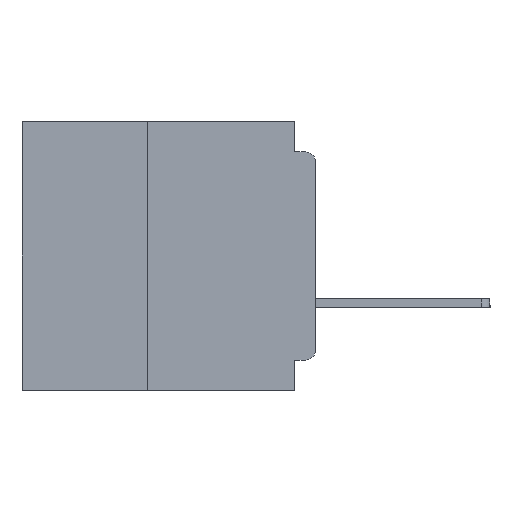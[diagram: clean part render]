
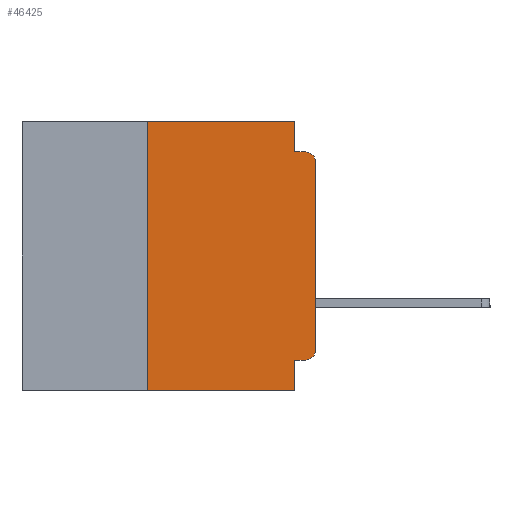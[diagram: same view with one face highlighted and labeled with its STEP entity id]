
A CAD part, left-side view. The second image highlights one B-rep face of the part: STEP entity #46425.
In plain terms, the highlighted planar face has unit normal (-1, 0, 0).
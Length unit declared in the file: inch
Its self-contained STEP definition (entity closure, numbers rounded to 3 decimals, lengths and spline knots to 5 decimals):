
#158 = VERTEX_POINT ( 'NONE', #44813 ) ;
#260 = ORIENTED_EDGE ( 'NONE', *, *, #31546, .T. ) ;
#1217 = CARTESIAN_POINT ( 'NONE',  ( 0., 0.437, 0. ) ) ;
#1366 = CARTESIAN_POINT ( 'NONE',  ( 0., 0., 0. ) ) ;
#1409 = DIRECTION ( 'NONE',  ( 0., 0., -1. ) ) ;
#1704 = VERTEX_POINT ( 'NONE', #16369 ) ;
#2099 = VECTOR ( 'NONE', #24303, 39.37008 ) ;
#3854 = VERTEX_POINT ( 'NONE', #15556 ) ;
#4200 = EDGE_CURVE ( 'NONE', #3854, #1704, #4926, .T. ) ;
#4202 = CARTESIAN_POINT ( 'NONE',  ( 0., 0.015, -0.06 ) ) ;
#4507 = DIRECTION ( 'NONE',  ( -1., 0., 0. ) ) ;
#4753 = DIRECTION ( 'NONE',  ( 0., 1., 0. ) ) ;
#4926 = LINE ( 'NONE', #34712, #16187 ) ;
#4936 = LINE ( 'NONE', #13848, #48570 ) ;
#5078 = CARTESIAN_POINT ( 'NONE',  ( 0., 0.015, -0.045 ) ) ;
#5503 = DIRECTION ( 'NONE',  ( 0., -1., 0. ) ) ;
#5647 = DIRECTION ( 'NONE',  ( 0., 0., 1. ) ) ;
#6201 = LINE ( 'NONE', #14201, #29228 ) ;
#7876 = VECTOR ( 'NONE', #4753, 39.37008 ) ;
#8481 = DIRECTION ( 'NONE',  ( 0., 0., -1. ) ) ;
#8859 = EDGE_CURVE ( 'NONE', #26395, #14210, #9221, .T. ) ;
#9221 = LINE ( 'NONE', #1366, #29024 ) ;
#9408 = DIRECTION ( 'NONE',  ( 0., 0., -1. ) ) ;
#10804 = CARTESIAN_POINT ( 'NONE',  ( 0., 0.25, -0.4 ) ) ;
#11711 = CARTESIAN_POINT ( 'NONE',  ( 0., 0., -0.045 ) ) ;
#11848 = AXIS2_PLACEMENT_3D ( 'NONE', #29822, #4507, #34080 ) ;
#12430 = CARTESIAN_POINT ( 'NONE',  ( 0., 0., -0.06 ) ) ;
#13848 = CARTESIAN_POINT ( 'NONE',  ( 0., 0.25, -0.4 ) ) ;
#14106 = CIRCLE ( 'NONE', #11848, 0.015 ) ;
#14201 = CARTESIAN_POINT ( 'NONE',  ( 0., 0.031, -0.4 ) ) ;
#14210 = VERTEX_POINT ( 'NONE', #12430 ) ;
#14764 = ORIENTED_EDGE ( 'NONE', *, *, #8859, .T. ) ;
#14933 = CARTESIAN_POINT ( 'NONE',  ( 0., 0.015, -0.355 ) ) ;
#14992 = CARTESIAN_POINT ( 'NONE',  ( 0., 0.25, 0. ) ) ;
#15556 = CARTESIAN_POINT ( 'NONE',  ( 0., 0.031, 0. ) ) ;
#16050 = LINE ( 'NONE', #20059, #2099 ) ;
#16174 = CARTESIAN_POINT ( 'NONE',  ( 0., 0.031, -0.4 ) ) ;
#16187 = VECTOR ( 'NONE', #9408, 39.37008 ) ;
#16284 = EDGE_CURVE ( 'NONE', #1704, #41318, #26384, .T. ) ;
#16369 = CARTESIAN_POINT ( 'NONE',  ( 0., 0.031, -0.045 ) ) ;
#18501 = ORIENTED_EDGE ( 'NONE', *, *, #45849, .T. ) ;
#19604 = EDGE_LOOP ( 'NONE', ( #14764, #18501, #52373, #53583, #40967, #48940, #43516, #31490, #33628, #260 ) ) ;
#20059 = CARTESIAN_POINT ( 'NONE',  ( 0., 0.437, -0.4 ) ) ;
#20092 = EDGE_CURVE ( 'NONE', #21934, #25555, #16050, .T. ) ;
#21934 = VERTEX_POINT ( 'NONE', #10804 ) ;
#24303 = DIRECTION ( 'NONE',  ( 0., -1., 0. ) ) ;
#25036 = DIRECTION ( 'NONE',  ( 1., 0., 0. ) ) ;
#25359 = CARTESIAN_POINT ( 'NONE',  ( 0., 0., -0.34 ) ) ;
#25555 = VERTEX_POINT ( 'NONE', #16174 ) ;
#26384 = LINE ( 'NONE', #11711, #48876 ) ;
#26395 = VERTEX_POINT ( 'NONE', #25359 ) ;
#27263 = EDGE_CURVE ( 'NONE', #158, #25555, #6201, .T. ) ;
#29024 = VECTOR ( 'NONE', #5647, 39.37008 ) ;
#29228 = VECTOR ( 'NONE', #1409, 39.37008 ) ;
#29389 = VECTOR ( 'NONE', #5503, 39.37008 ) ;
#29822 = CARTESIAN_POINT ( 'NONE',  ( 0., 0.015, -0.34 ) ) ;
#30062 = CARTESIAN_POINT ( 'NONE',  ( 0., 0., -0.355 ) ) ;
#30360 = LINE ( 'NONE', #30062, #7876 ) ;
#31490 = ORIENTED_EDGE ( 'NONE', *, *, #27263, .F. ) ;
#31546 = EDGE_CURVE ( 'NONE', #51171, #26395, #14106, .T. ) ;
#33356 = PLANE ( 'NONE',  #49285 ) ;
#33628 = ORIENTED_EDGE ( 'NONE', *, *, #39635, .F. ) ;
#33792 = DIRECTION ( 'NONE',  ( -1., 0., 0. ) ) ;
#34080 = DIRECTION ( 'NONE',  ( 0., 0., -1. ) ) ;
#34712 = CARTESIAN_POINT ( 'NONE',  ( 0., 0.031, 0. ) ) ;
#36928 = EDGE_CURVE ( 'NONE', #21934, #42175, #4936, .T. ) ;
#37226 = AXIS2_PLACEMENT_3D ( 'NONE', #4202, #33792, #8481 ) ;
#39177 = DIRECTION ( 'NONE',  ( 0., 0., 1. ) ) ;
#39635 = EDGE_CURVE ( 'NONE', #51171, #158, #30360, .T. ) ;
#40967 = ORIENTED_EDGE ( 'NONE', *, *, #42661, .F. ) ;
#41318 = VERTEX_POINT ( 'NONE', #5078 ) ;
#41332 = FACE_OUTER_BOUND ( 'NONE', #19604, .T. ) ;
#42175 = VERTEX_POINT ( 'NONE', #14992 ) ;
#42661 = EDGE_CURVE ( 'NONE', #42175, #3854, #51933, .T. ) ;
#43516 = ORIENTED_EDGE ( 'NONE', *, *, #20092, .T. ) ;
#44813 = CARTESIAN_POINT ( 'NONE',  ( 0., 0.031, -0.355 ) ) ;
#45849 = EDGE_CURVE ( 'NONE', #14210, #41318, #49349, .T. ) ;
#46425 = ADVANCED_FACE ( 'NONE', ( #41332 ), #33356, .F. ) ;
#48570 = VECTOR ( 'NONE', #39177, 39.37008 ) ;
#48876 = VECTOR ( 'NONE', #49627, 39.37008 ) ;
#48940 = ORIENTED_EDGE ( 'NONE', *, *, #36928, .F. ) ;
#49285 = AXIS2_PLACEMENT_3D ( 'NONE', #50399, #25036, #54637 ) ;
#49349 = CIRCLE ( 'NONE', #37226, 0.015 ) ;
#49627 = DIRECTION ( 'NONE',  ( 0., -1., 0. ) ) ;
#50399 = CARTESIAN_POINT ( 'NONE',  ( 0., 0.437, 0. ) ) ;
#51171 = VERTEX_POINT ( 'NONE', #14933 ) ;
#51933 = LINE ( 'NONE', #1217, #29389 ) ;
#52373 = ORIENTED_EDGE ( 'NONE', *, *, #16284, .F. ) ;
#53583 = ORIENTED_EDGE ( 'NONE', *, *, #4200, .F. ) ;
#54637 = DIRECTION ( 'NONE',  ( 0., 0., -1. ) ) ;
